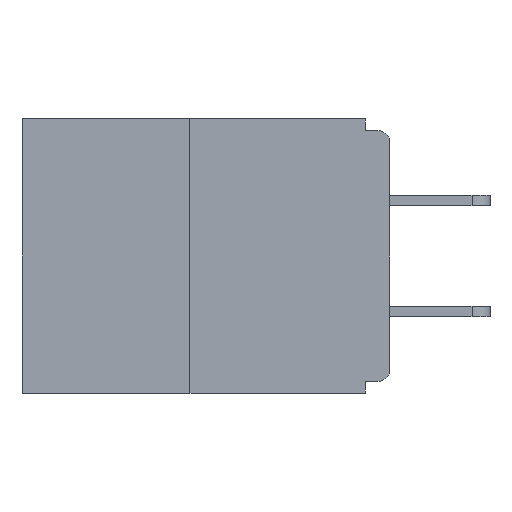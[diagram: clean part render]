
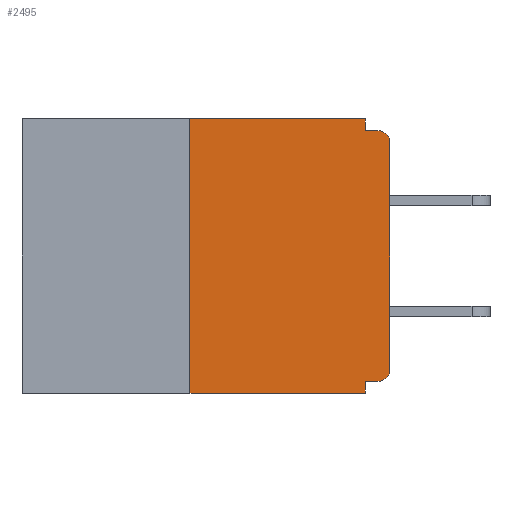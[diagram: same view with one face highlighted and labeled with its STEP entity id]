
A CAD part, left-side view. The second image highlights one B-rep face of the part: STEP entity #2495.
In plain terms, the highlighted planar face has unit normal (-1, 0, 0).
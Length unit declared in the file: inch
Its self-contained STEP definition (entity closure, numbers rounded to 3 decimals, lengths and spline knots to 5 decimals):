
#523 = ORIENTED_EDGE ( 'NONE', *, *, #19121, .F. ) ;
#2128 = DIRECTION ( 'NONE',  ( 0., -1., 0. ) ) ;
#2310 = VERTEX_POINT ( 'NONE', #16901 ) ;
#2463 = ORIENTED_EDGE ( 'NONE', *, *, #22659, .F. ) ;
#2495 = ADVANCED_FACE ( 'NONE', ( #16717 ), #21819, .F. ) ;
#3342 = VERTEX_POINT ( 'NONE', #7225 ) ;
#3362 = VECTOR ( 'NONE', #17615, 39.37008 ) ;
#3384 = LINE ( 'NONE', #11356, #20493 ) ;
#3701 = DIRECTION ( 'NONE',  ( 0., 0., -1. ) ) ;
#3845 = CARTESIAN_POINT ( 'NONE',  ( 0., 0.015, -0.03 ) ) ;
#3883 = CIRCLE ( 'NONE', #7451, 0.015 ) ;
#4283 = DIRECTION ( 'NONE',  ( 0., -1., 0. ) ) ;
#4293 = CARTESIAN_POINT ( 'NONE',  ( 0., 0.031, -0.343 ) ) ;
#4399 = VERTEX_POINT ( 'NONE', #11365 ) ;
#4455 = VERTEX_POINT ( 'NONE', #19146 ) ;
#4991 = LINE ( 'NONE', #11229, #15349 ) ;
#5111 = DIRECTION ( 'NONE',  ( 0., 0., 1. ) ) ;
#5249 = EDGE_CURVE ( 'NONE', #22975, #21879, #3384, .T. ) ;
#5589 = DIRECTION ( 'NONE',  ( 1., 0., 0. ) ) ;
#5623 = LINE ( 'NONE', #4293, #3362 ) ;
#5869 = ORIENTED_EDGE ( 'NONE', *, *, #21881, .T. ) ;
#6223 = CARTESIAN_POINT ( 'NONE',  ( 0., 0., -0.328 ) ) ;
#6433 = EDGE_CURVE ( 'NONE', #2310, #21879, #3883, .T. ) ;
#6570 = CARTESIAN_POINT ( 'NONE',  ( 0., 0.015, -0.328 ) ) ;
#6631 = CARTESIAN_POINT ( 'NONE',  ( 0., 0.031, 0. ) ) ;
#6637 = LINE ( 'NONE', #8091, #9729 ) ;
#6850 = CARTESIAN_POINT ( 'NONE',  ( 0., 0.031, 0. ) ) ;
#7106 = EDGE_CURVE ( 'NONE', #16763, #22975, #11964, .T. ) ;
#7124 = ORIENTED_EDGE ( 'NONE', *, *, #5249, .F. ) ;
#7225 = CARTESIAN_POINT ( 'NONE',  ( 0., 0.031, -0.343 ) ) ;
#7451 = AXIS2_PLACEMENT_3D ( 'NONE', #3845, #13183, #11532 ) ;
#7567 = EDGE_CURVE ( 'NONE', #17335, #3342, #5623, .T. ) ;
#7841 = DIRECTION ( 'NONE',  ( 0., 1., 0. ) ) ;
#8091 = CARTESIAN_POINT ( 'NONE',  ( 0., 0., 0. ) ) ;
#8774 = EDGE_CURVE ( 'NONE', #4455, #3342, #4991, .T. ) ;
#9315 = EDGE_LOOP ( 'NONE', ( #523, #10961, #19072, #19570, #2463, #20906, #5869, #19859, #7124, #11488 ) ) ;
#9729 = VECTOR ( 'NONE', #11719, 39.37008 ) ;
#9803 = CARTESIAN_POINT ( 'NONE',  ( 0., 0.015, -0.313 ) ) ;
#10528 = CARTESIAN_POINT ( 'NONE',  ( 0., 0.031, -0.328 ) ) ;
#10961 = ORIENTED_EDGE ( 'NONE', *, *, #21208, .F. ) ;
#11229 = CARTESIAN_POINT ( 'NONE',  ( 0., 0.46, -0.343 ) ) ;
#11293 = DIRECTION ( 'NONE',  ( 0., 0., -1. ) ) ;
#11356 = CARTESIAN_POINT ( 'NONE',  ( 0., 0., -0.015 ) ) ;
#11365 = CARTESIAN_POINT ( 'NONE',  ( 0., 0., -0.313 ) ) ;
#11488 = ORIENTED_EDGE ( 'NONE', *, *, #7106, .F. ) ;
#11532 = DIRECTION ( 'NONE',  ( 0., 0., -1. ) ) ;
#11637 = VECTOR ( 'NONE', #7841, 39.37008 ) ;
#11719 = DIRECTION ( 'NONE',  ( 0., 0., 1. ) ) ;
#11964 = LINE ( 'NONE', #6631, #12547 ) ;
#12547 = VECTOR ( 'NONE', #13832, 39.37008 ) ;
#12649 = CARTESIAN_POINT ( 'NONE',  ( 0., 0.25, 0. ) ) ;
#13183 = DIRECTION ( 'NONE',  ( -1., 0., 0. ) ) ;
#13229 = EDGE_CURVE ( 'NONE', #21674, #4399, #21345, .T. ) ;
#13832 = DIRECTION ( 'NONE',  ( 0., 0., -1. ) ) ;
#14055 = DIRECTION ( 'NONE',  ( 0., -1., 0. ) ) ;
#14153 = VERTEX_POINT ( 'NONE', #12649 ) ;
#15349 = VECTOR ( 'NONE', #2128, 39.37008 ) ;
#15896 = CARTESIAN_POINT ( 'NONE',  ( 0., 0.031, -0.015 ) ) ;
#16210 = LINE ( 'NONE', #17578, #21826 ) ;
#16717 = FACE_OUTER_BOUND ( 'NONE', #9315, .T. ) ;
#16763 = VERTEX_POINT ( 'NONE', #6850 ) ;
#16901 = CARTESIAN_POINT ( 'NONE',  ( 0., 0., -0.03 ) ) ;
#17335 = VERTEX_POINT ( 'NONE', #10528 ) ;
#17578 = CARTESIAN_POINT ( 'NONE',  ( 0., 0.25, 0. ) ) ;
#17615 = DIRECTION ( 'NONE',  ( 0., 0., -1. ) ) ;
#17777 = AXIS2_PLACEMENT_3D ( 'NONE', #17968, #5589, #3701 ) ;
#17968 = CARTESIAN_POINT ( 'NONE',  ( 0., 0.46, 0. ) ) ;
#18587 = VECTOR ( 'NONE', #14055, 39.37008 ) ;
#19072 = ORIENTED_EDGE ( 'NONE', *, *, #8774, .T. ) ;
#19121 = EDGE_CURVE ( 'NONE', #14153, #16763, #20563, .T. ) ;
#19146 = CARTESIAN_POINT ( 'NONE',  ( 0., 0.25, -0.343 ) ) ;
#19168 = AXIS2_PLACEMENT_3D ( 'NONE', #9803, #22329, #11293 ) ;
#19570 = ORIENTED_EDGE ( 'NONE', *, *, #7567, .F. ) ;
#19859 = ORIENTED_EDGE ( 'NONE', *, *, #6433, .T. ) ;
#20104 = CARTESIAN_POINT ( 'NONE',  ( 0., 0.46, 0. ) ) ;
#20493 = VECTOR ( 'NONE', #4283, 39.37008 ) ;
#20563 = LINE ( 'NONE', #20104, #18587 ) ;
#20906 = ORIENTED_EDGE ( 'NONE', *, *, #13229, .T. ) ;
#21208 = EDGE_CURVE ( 'NONE', #4455, #14153, #16210, .T. ) ;
#21345 = CIRCLE ( 'NONE', #19168, 0.015 ) ;
#21674 = VERTEX_POINT ( 'NONE', #6570 ) ;
#21819 = PLANE ( 'NONE',  #17777 ) ;
#21826 = VECTOR ( 'NONE', #5111, 39.37008 ) ;
#21879 = VERTEX_POINT ( 'NONE', #22246 ) ;
#21881 = EDGE_CURVE ( 'NONE', #4399, #2310, #6637, .T. ) ;
#22246 = CARTESIAN_POINT ( 'NONE',  ( 0., 0.015, -0.015 ) ) ;
#22299 = LINE ( 'NONE', #6223, #11637 ) ;
#22329 = DIRECTION ( 'NONE',  ( -1., 0., 0. ) ) ;
#22659 = EDGE_CURVE ( 'NONE', #21674, #17335, #22299, .T. ) ;
#22975 = VERTEX_POINT ( 'NONE', #15896 ) ;
